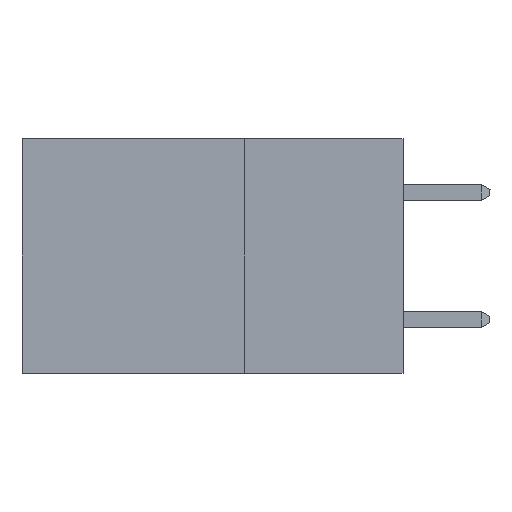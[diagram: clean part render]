
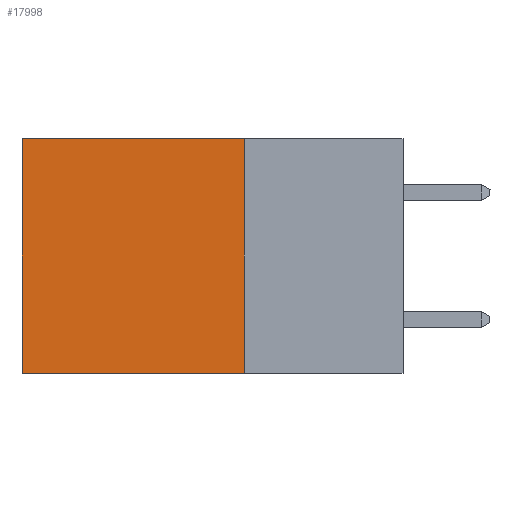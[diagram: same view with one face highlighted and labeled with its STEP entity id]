
A CAD part, left-side view. The second image highlights one B-rep face of the part: STEP entity #17998.
In plain terms, the highlighted planar face has unit normal (-1, 0, 0).
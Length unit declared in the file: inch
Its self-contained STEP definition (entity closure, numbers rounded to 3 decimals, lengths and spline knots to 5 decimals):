
#286 = CARTESIAN_POINT ( 'NONE',  ( 0.2875, 0.25, 0. ) ) ;
#722 = LINE ( 'NONE', #24164, #6831 ) ;
#1747 = DIRECTION ( 'NONE',  ( 0., 1., 0. ) ) ;
#2108 = AXIS2_PLACEMENT_3D ( 'NONE', #19443, #13428, #19593 ) ;
#4600 = DIRECTION ( 'NONE',  ( 0., 0., -1. ) ) ;
#4748 = CARTESIAN_POINT ( 'NONE',  ( 0.2875, 0.25, -0.37 ) ) ;
#4813 = EDGE_CURVE ( 'NONE', #19622, #16875, #25133, .T. ) ;
#6003 = EDGE_CURVE ( 'NONE', #21221, #19622, #722, .T. ) ;
#6831 = VECTOR ( 'NONE', #13569, 39.37008 ) ;
#7595 = DIRECTION ( 'NONE',  ( 0., 0., -1. ) ) ;
#8119 = ORIENTED_EDGE ( 'NONE', *, *, #17183, .F. ) ;
#8748 = PLANE ( 'NONE',  #2108 ) ;
#9759 = EDGE_CURVE ( 'NONE', #21221, #26390, #24029, .T. ) ;
#10734 = EDGE_LOOP ( 'NONE', ( #20121, #8119, #18399, #27793 ) ) ;
#10839 = CARTESIAN_POINT ( 'NONE',  ( 0.2875, 0.25, -0.37 ) ) ;
#11203 = VECTOR ( 'NONE', #1747, 39.37008 ) ;
#11307 = FACE_OUTER_BOUND ( 'NONE', #10734, .T. ) ;
#11857 = CARTESIAN_POINT ( 'NONE',  ( 0.2875, 0.6, 0. ) ) ;
#13428 = DIRECTION ( 'NONE',  ( 1., 0., 0. ) ) ;
#13569 = DIRECTION ( 'NONE',  ( 0., 1., 0. ) ) ;
#13577 = CARTESIAN_POINT ( 'NONE',  ( 0.2875, 0.25, 0. ) ) ;
#13702 = CARTESIAN_POINT ( 'NONE',  ( 0.2875, 0.6, -0.37 ) ) ;
#14175 = VECTOR ( 'NONE', #4600, 39.37008 ) ;
#16875 = VERTEX_POINT ( 'NONE', #13702 ) ;
#17183 = EDGE_CURVE ( 'NONE', #26390, #16875, #21551, .T. ) ;
#17998 = ADVANCED_FACE ( 'NONE', ( #11307 ), #8748, .F. ) ;
#18399 = ORIENTED_EDGE ( 'NONE', *, *, #9759, .F. ) ;
#19443 = CARTESIAN_POINT ( 'NONE',  ( 0.2875, 0.25, 0. ) ) ;
#19593 = DIRECTION ( 'NONE',  ( 0., 0., -1. ) ) ;
#19622 = VERTEX_POINT ( 'NONE', #27854 ) ;
#20121 = ORIENTED_EDGE ( 'NONE', *, *, #4813, .T. ) ;
#21221 = VERTEX_POINT ( 'NONE', #286 ) ;
#21551 = LINE ( 'NONE', #10839, #11203 ) ;
#24029 = LINE ( 'NONE', #13577, #14175 ) ;
#24164 = CARTESIAN_POINT ( 'NONE',  ( 0.2875, 0.25, 0. ) ) ;
#24495 = VECTOR ( 'NONE', #7595, 39.37008 ) ;
#25133 = LINE ( 'NONE', #11857, #24495 ) ;
#26390 = VERTEX_POINT ( 'NONE', #4748 ) ;
#27793 = ORIENTED_EDGE ( 'NONE', *, *, #6003, .T. ) ;
#27854 = CARTESIAN_POINT ( 'NONE',  ( 0.2875, 0.6, 0. ) ) ;
